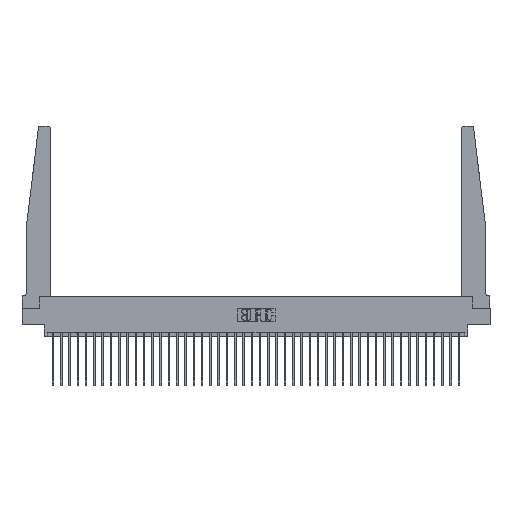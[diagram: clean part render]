
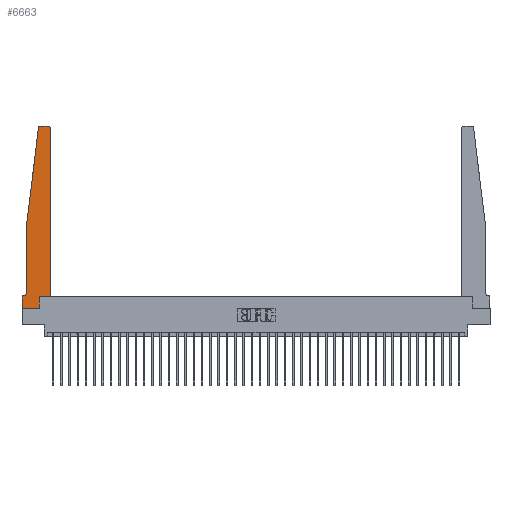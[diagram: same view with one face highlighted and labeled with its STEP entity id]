
A CAD part, top view. The second image highlights one B-rep face of the part: STEP entity #6663.
In plain terms, the highlighted planar face has unit normal (0, 0, 1).
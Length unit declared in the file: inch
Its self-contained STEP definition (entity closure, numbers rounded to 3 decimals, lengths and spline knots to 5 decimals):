
#45 = VERTEX_POINT ( 'NONE', #7064 ) ;
#1013 = VERTEX_POINT ( 'NONE', #4722 ) ;
#1018 = EDGE_CURVE ( 'NONE', #2881, #17520, #25263, .T. ) ;
#1122 = CARTESIAN_POINT ( 'NONE',  ( 0.015, 0.1875, 0.37 ) ) ;
#1194 = ORIENTED_EDGE ( 'NONE', *, *, #24279, .T. ) ;
#1717 = EDGE_CURVE ( 'NONE', #9840, #27966, #19369, .T. ) ;
#1852 = DIRECTION ( 'NONE',  ( 1., 0., 0. ) ) ;
#2386 = EDGE_CURVE ( 'NONE', #1013, #31751, #12923, .T. ) ;
#2630 = EDGE_CURVE ( 'NONE', #36122, #9840, #26510, .T. ) ;
#2739 = CARTESIAN_POINT ( 'NONE',  ( 0.25, 2.75, 0.37 ) ) ;
#2828 = CARTESIAN_POINT ( 'NONE',  ( 0., 0., 0.37 ) ) ;
#2881 = VERTEX_POINT ( 'NONE', #30589 ) ;
#3351 = AXIS2_PLACEMENT_3D ( 'NONE', #12435, #23993, #26445 ) ;
#4722 = CARTESIAN_POINT ( 'NONE',  ( 0.2605, 0.18, 0.37 ) ) ;
#5110 = CARTESIAN_POINT ( 'NONE',  ( 0.395, 2.75, 0.37 ) ) ;
#5204 = CARTESIAN_POINT ( 'NONE',  ( 0.27653, 2.75, 0.37 ) ) ;
#5445 = VECTOR ( 'NONE', #29032, 39.37008 ) ;
#5721 = LINE ( 'NONE', #11735, #22877 ) ;
#5725 = DIRECTION ( 'NONE',  ( 1., 0., 0. ) ) ;
#6663 = ADVANCED_FACE ( 'NONE', ( #32043 ), #26265, .T. ) ;
#7064 = CARTESIAN_POINT ( 'NONE',  ( 0.425, 2.72, 0.37 ) ) ;
#7305 = AXIS2_PLACEMENT_3D ( 'NONE', #31831, #8844, #27095 ) ;
#7532 = EDGE_CURVE ( 'NONE', #17520, #36122, #17767, .T. ) ;
#8045 = LINE ( 'NONE', #30854, #12087 ) ;
#8401 = EDGE_CURVE ( 'NONE', #14442, #2881, #18902, .T. ) ;
#8844 = DIRECTION ( 'NONE',  ( 0., 0., 1. ) ) ;
#9301 = CIRCLE ( 'NONE', #33757, 0.03 ) ;
#9840 = VERTEX_POINT ( 'NONE', #25513 ) ;
#9849 = CARTESIAN_POINT ( 'NONE',  ( 0.015, 0.2375, 0.37 ) ) ;
#10254 = ORIENTED_EDGE ( 'NONE', *, *, #16171, .T. ) ;
#10521 = ORIENTED_EDGE ( 'NONE', *, *, #10770, .T. ) ;
#10770 = EDGE_CURVE ( 'NONE', #27966, #23381, #33841, .T. ) ;
#10984 = DIRECTION ( 'NONE',  ( 0., 0., 1. ) ) ;
#11261 = CARTESIAN_POINT ( 'NONE',  ( 0.425, 0.18, 0.37 ) ) ;
#11735 = CARTESIAN_POINT ( 'NONE',  ( 0.425, 0.18, 0.37 ) ) ;
#12087 = VECTOR ( 'NONE', #31027, 39.37008 ) ;
#12131 = CARTESIAN_POINT ( 'NONE',  ( 0.065, 0.1875, 0.37 ) ) ;
#12435 = CARTESIAN_POINT ( 'NONE',  ( 0., 0.1875, 0.37 ) ) ;
#12915 = ORIENTED_EDGE ( 'NONE', *, *, #30350, .T. ) ;
#12923 = LINE ( 'NONE', #30636, #35120 ) ;
#14149 = DIRECTION ( 'NONE',  ( -1., 0., 0. ) ) ;
#14442 = VERTEX_POINT ( 'NONE', #19413 ) ;
#15515 = DIRECTION ( 'NONE',  ( 1., 0., 0. ) ) ;
#15758 = ORIENTED_EDGE ( 'NONE', *, *, #2630, .T. ) ;
#15817 = EDGE_LOOP ( 'NONE', ( #26666, #22227, #26007, #22038, #23656, #15758, #32465, #10521, #12915, #35623, #10254, #1194 ) ) ;
#16171 = EDGE_CURVE ( 'NONE', #31751, #45, #5721, .T. ) ;
#17473 = CIRCLE ( 'NONE', #7305, 0.03 ) ;
#17520 = VERTEX_POINT ( 'NONE', #21933 ) ;
#17645 = CARTESIAN_POINT ( 'NONE',  ( 0., 0., 0.37 ) ) ;
#17767 = CIRCLE ( 'NONE', #20741, 0.05 ) ;
#18307 = VECTOR ( 'NONE', #36116, 39.37008 ) ;
#18902 = LINE ( 'NONE', #24880, #18307 ) ;
#19369 = LINE ( 'NONE', #17645, #5445 ) ;
#19413 = CARTESIAN_POINT ( 'NONE',  ( 0.24675, 2.72367, 0.37 ) ) ;
#19733 = LINE ( 'NONE', #2739, #32986 ) ;
#20741 = AXIS2_PLACEMENT_3D ( 'NONE', #9849, #27218, #21242 ) ;
#21242 = DIRECTION ( 'NONE',  ( -1., 0., 0. ) ) ;
#21260 = CARTESIAN_POINT ( 'NONE',  ( 0., 0., 0.37 ) ) ;
#21746 = VECTOR ( 'NONE', #15515, 39.37008 ) ;
#21933 = CARTESIAN_POINT ( 'NONE',  ( 0.065, 0.2375, 0.37 ) ) ;
#22038 = ORIENTED_EDGE ( 'NONE', *, *, #1018, .T. ) ;
#22151 = VECTOR ( 'NONE', #22643, 39.37008 ) ;
#22227 = ORIENTED_EDGE ( 'NONE', *, *, #33940, .T. ) ;
#22643 = DIRECTION ( 'NONE',  ( 0., -1., 0. ) ) ;
#22877 = VECTOR ( 'NONE', #23091, 39.37008 ) ;
#23091 = DIRECTION ( 'NONE',  ( 0., 1., 0. ) ) ;
#23381 = VERTEX_POINT ( 'NONE', #26681 ) ;
#23656 = ORIENTED_EDGE ( 'NONE', *, *, #7532, .T. ) ;
#23993 = DIRECTION ( 'NONE',  ( 0., 0., 1. ) ) ;
#24279 = EDGE_CURVE ( 'NONE', #45, #31150, #17473, .T. ) ;
#24513 = VERTEX_POINT ( 'NONE', #5204 ) ;
#24880 = CARTESIAN_POINT ( 'NONE',  ( 0.065, 1.25, 0.37 ) ) ;
#25263 = LINE ( 'NONE', #36322, #22151 ) ;
#25513 = CARTESIAN_POINT ( 'NONE',  ( 0., 0.1875, 0.37 ) ) ;
#26007 = ORIENTED_EDGE ( 'NONE', *, *, #8401, .T. ) ;
#26265 = PLANE ( 'NONE',  #3351 ) ;
#26445 = DIRECTION ( 'NONE',  ( 1., 0., 0. ) ) ;
#26510 = LINE ( 'NONE', #12131, #32736 ) ;
#26666 = ORIENTED_EDGE ( 'NONE', *, *, #30891, .T. ) ;
#26681 = CARTESIAN_POINT ( 'NONE',  ( 0.2605, 0., 0.37 ) ) ;
#27095 = DIRECTION ( 'NONE',  ( 1., 0., 0. ) ) ;
#27218 = DIRECTION ( 'NONE',  ( 0., 0., -1. ) ) ;
#27966 = VERTEX_POINT ( 'NONE', #21260 ) ;
#28708 = CARTESIAN_POINT ( 'NONE',  ( 0.27653, 2.72, 0.37 ) ) ;
#29032 = DIRECTION ( 'NONE',  ( 0., -1., 0. ) ) ;
#30350 = EDGE_CURVE ( 'NONE', #23381, #1013, #8045, .T. ) ;
#30589 = CARTESIAN_POINT ( 'NONE',  ( 0.065, 1.25, 0.37 ) ) ;
#30636 = CARTESIAN_POINT ( 'NONE',  ( 0.425, 0.18, 0.37 ) ) ;
#30854 = CARTESIAN_POINT ( 'NONE',  ( 0.2605, 0.18, 0.37 ) ) ;
#30891 = EDGE_CURVE ( 'NONE', #31150, #24513, #19733, .T. ) ;
#31027 = DIRECTION ( 'NONE',  ( 0., 1., 0. ) ) ;
#31150 = VERTEX_POINT ( 'NONE', #5110 ) ;
#31751 = VERTEX_POINT ( 'NONE', #11261 ) ;
#31831 = CARTESIAN_POINT ( 'NONE',  ( 0.395, 2.72, 0.37 ) ) ;
#32043 = FACE_OUTER_BOUND ( 'NONE', #15817, .T. ) ;
#32465 = ORIENTED_EDGE ( 'NONE', *, *, #1717, .T. ) ;
#32736 = VECTOR ( 'NONE', #35292, 39.37008 ) ;
#32986 = VECTOR ( 'NONE', #14149, 39.37008 ) ;
#33757 = AXIS2_PLACEMENT_3D ( 'NONE', #28708, #10984, #5725 ) ;
#33841 = LINE ( 'NONE', #2828, #21746 ) ;
#33940 = EDGE_CURVE ( 'NONE', #24513, #14442, #9301, .T. ) ;
#35120 = VECTOR ( 'NONE', #1852, 39.37008 ) ;
#35292 = DIRECTION ( 'NONE',  ( -1., 0., 0. ) ) ;
#35623 = ORIENTED_EDGE ( 'NONE', *, *, #2386, .T. ) ;
#36116 = DIRECTION ( 'NONE',  ( -0.122, -0.992, 0. ) ) ;
#36122 = VERTEX_POINT ( 'NONE', #1122 ) ;
#36322 = CARTESIAN_POINT ( 'NONE',  ( 0.065, 1.25, 0.37 ) ) ;
